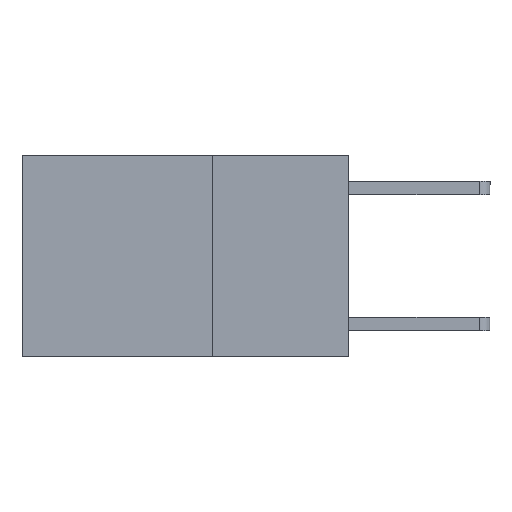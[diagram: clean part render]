
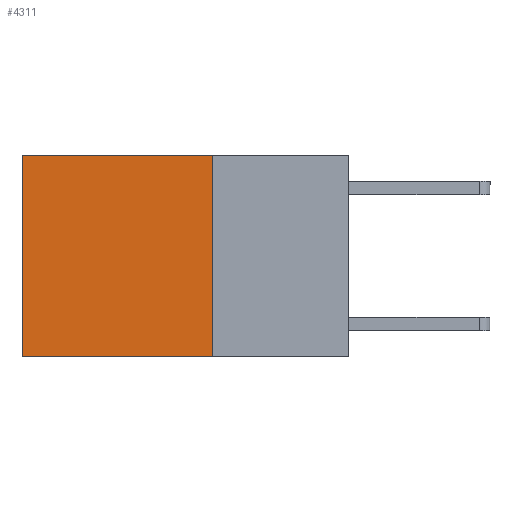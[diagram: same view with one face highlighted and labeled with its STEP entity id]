
A CAD part, left-side view. The second image highlights one B-rep face of the part: STEP entity #4311.
In plain terms, the highlighted planar face has unit normal (-1, 0, 0).
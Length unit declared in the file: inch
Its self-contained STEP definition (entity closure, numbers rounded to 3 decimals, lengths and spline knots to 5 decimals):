
#29 = LINE ( 'NONE', #1934, #2363 ) ;
#271 = EDGE_CURVE ( 'NONE', #5817, #6396, #7520, .T. ) ;
#307 = EDGE_CURVE ( 'NONE', #5871, #4702, #29, .T. ) ;
#756 = CARTESIAN_POINT ( 'NONE',  ( 0.2625, 0.6, -0.37 ) ) ;
#1151 = ORIENTED_EDGE ( 'NONE', *, *, #1277, .F. ) ;
#1277 = EDGE_CURVE ( 'NONE', #4702, #6396, #4998, .T. ) ;
#1867 = DIRECTION ( 'NONE',  ( 0., 1., 0. ) ) ;
#1934 = CARTESIAN_POINT ( 'NONE',  ( 0.2625, 0.25, 0. ) ) ;
#2265 = ORIENTED_EDGE ( 'NONE', *, *, #2843, .T. ) ;
#2267 = AXIS2_PLACEMENT_3D ( 'NONE', #3376, #6964, #3953 ) ;
#2363 = VECTOR ( 'NONE', #5560, 39.37008 ) ;
#2394 = CARTESIAN_POINT ( 'NONE',  ( 0.2625, 0.6, 0. ) ) ;
#2634 = DIRECTION ( 'NONE',  ( 0., 1., 0. ) ) ;
#2843 = EDGE_CURVE ( 'NONE', #5871, #5817, #3809, .T. ) ;
#3376 = CARTESIAN_POINT ( 'NONE',  ( 0.2625, 0.25, 0. ) ) ;
#3804 = DIRECTION ( 'NONE',  ( 0., 0., -1. ) ) ;
#3809 = LINE ( 'NONE', #4462, #5738 ) ;
#3878 = FACE_OUTER_BOUND ( 'NONE', #6343, .T. ) ;
#3943 = CARTESIAN_POINT ( 'NONE',  ( 0.2625, 0.25, -0.37 ) ) ;
#3953 = DIRECTION ( 'NONE',  ( 0., 0., -1. ) ) ;
#4311 = ADVANCED_FACE ( 'NONE', ( #3878 ), #5172, .F. ) ;
#4462 = CARTESIAN_POINT ( 'NONE',  ( 0.2625, 0.25, 0. ) ) ;
#4702 = VERTEX_POINT ( 'NONE', #3943 ) ;
#4819 = CARTESIAN_POINT ( 'NONE',  ( 0.2625, 0.6, 0. ) ) ;
#4864 = CARTESIAN_POINT ( 'NONE',  ( 0.2625, 0.25, 0. ) ) ;
#4995 = ORIENTED_EDGE ( 'NONE', *, *, #271, .T. ) ;
#4998 = LINE ( 'NONE', #6253, #7980 ) ;
#5172 = PLANE ( 'NONE',  #2267 ) ;
#5560 = DIRECTION ( 'NONE',  ( 0., 0., -1. ) ) ;
#5738 = VECTOR ( 'NONE', #2634, 39.37008 ) ;
#5817 = VERTEX_POINT ( 'NONE', #4819 ) ;
#5871 = VERTEX_POINT ( 'NONE', #4864 ) ;
#6253 = CARTESIAN_POINT ( 'NONE',  ( 0.2625, 0.25, -0.37 ) ) ;
#6343 = EDGE_LOOP ( 'NONE', ( #4995, #1151, #7297, #2265 ) ) ;
#6396 = VERTEX_POINT ( 'NONE', #756 ) ;
#6964 = DIRECTION ( 'NONE',  ( 1., 0., 0. ) ) ;
#7103 = VECTOR ( 'NONE', #3804, 39.37008 ) ;
#7297 = ORIENTED_EDGE ( 'NONE', *, *, #307, .F. ) ;
#7520 = LINE ( 'NONE', #2394, #7103 ) ;
#7980 = VECTOR ( 'NONE', #1867, 39.37008 ) ;
